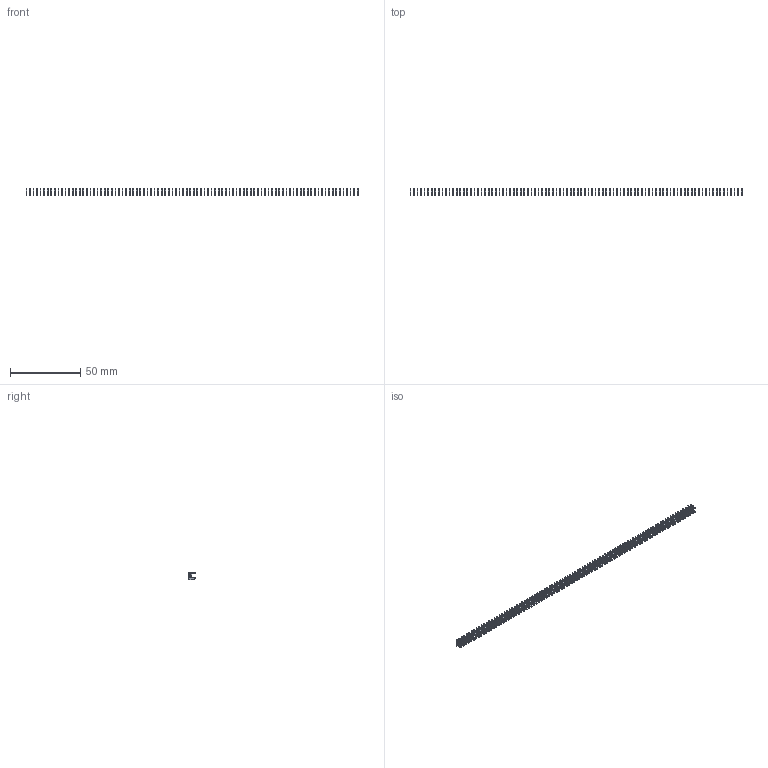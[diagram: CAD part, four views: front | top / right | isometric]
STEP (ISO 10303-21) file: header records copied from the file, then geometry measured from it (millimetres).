
FILE_DESCRIPTION (( 'STEP AP203' ), '1' );
FILE_NAME ('105-094-208-100.STEP', '2020-04-08T01:14:40', ( '' ), ( '' ), 'SwSTEP 2.0', 'SolidWorks 2016', '' );
FILE_SCHEMA (( 'CONFIG_CONTROL_DESIGN' ));
Length unit declared in the file: inch
Products named in the file (2): 100-290-001_100-290-208; 105-094-208-100
Assembly tree (94 placements, depth 2):
  105-094-208-100
    100-290-001_100-290-208  x94
Bounding box: 236.73 x 4.82 x 5.17 mm (x, y, z)
Volume: 646.8 mm3; surface area: 3994.6 mm2
Topology: 94 solids, 94 shells, 2350 faces, 6486 edges, 4324 vertices
Faces by surface type: plane 2068, cylinder 282
Entity records: 3965 total; most frequent: DIRECTION 319, CARTESIAN_POINT 237, DATE_AND_TIME 198, COORDINATED_UNIVERSAL_TIME_OFFSET 198, CALENDAR_DATE 198, LOCAL_TIME 198, ORIENTED_EDGE 138, AXIS2_PLACEMENT_3D 128
